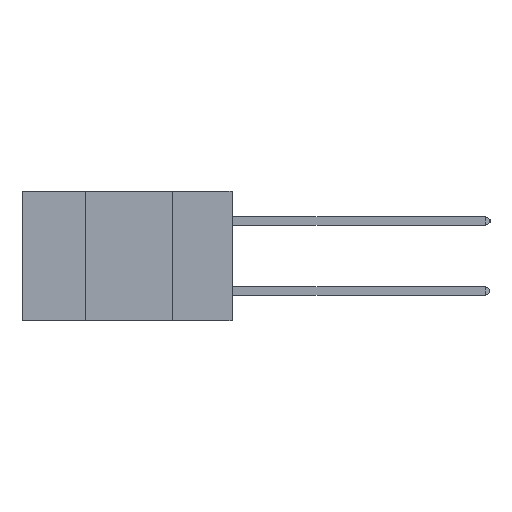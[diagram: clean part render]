
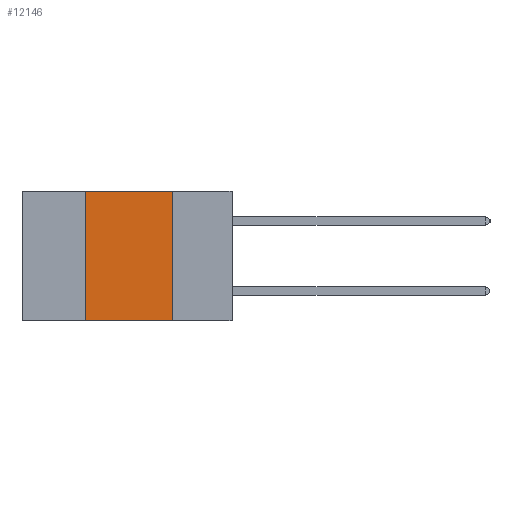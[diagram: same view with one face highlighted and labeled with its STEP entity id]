
A CAD part, left-side view. The second image highlights one B-rep face of the part: STEP entity #12146.
In plain terms, the highlighted planar face has unit normal (-1, 0, 0).
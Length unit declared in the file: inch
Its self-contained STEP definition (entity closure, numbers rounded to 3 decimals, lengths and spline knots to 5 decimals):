
#1187 = VECTOR ( 'NONE', #5307, 39.37008 ) ;
#1372 = ORIENTED_EDGE ( 'NONE', *, *, #10143, .F. ) ;
#1518 = EDGE_LOOP ( 'NONE', ( #11757, #1372, #4082, #6726 ) ) ;
#1736 = DIRECTION ( 'NONE',  ( 1., 0., 0. ) ) ;
#1915 = VERTEX_POINT ( 'NONE', #3395 ) ;
#2028 = CARTESIAN_POINT ( 'NONE',  ( 0., 0.6, -0.37 ) ) ;
#2125 = EDGE_CURVE ( 'NONE', #6571, #8781, #4030, .T. ) ;
#2692 = CARTESIAN_POINT ( 'NONE',  ( 0., 0.17, -0.37 ) ) ;
#2729 = DIRECTION ( 'NONE',  ( 0., 0., 1. ) ) ;
#2883 = CARTESIAN_POINT ( 'NONE',  ( 0., 0.42, 0. ) ) ;
#3104 = AXIS2_PLACEMENT_3D ( 'NONE', #11746, #1736, #8810 ) ;
#3157 = CARTESIAN_POINT ( 'NONE',  ( 0., 0.17, 0. ) ) ;
#3200 = DIRECTION ( 'NONE',  ( 0., 0., -1. ) ) ;
#3228 = CARTESIAN_POINT ( 'NONE',  ( 0., 0.42, -0.37 ) ) ;
#3395 = CARTESIAN_POINT ( 'NONE',  ( 0., 0.42, 0. ) ) ;
#3723 = VECTOR ( 'NONE', #11494, 39.37008 ) ;
#3902 = LINE ( 'NONE', #2883, #11580 ) ;
#4030 = LINE ( 'NONE', #2028, #3723 ) ;
#4082 = ORIENTED_EDGE ( 'NONE', *, *, #5499, .F. ) ;
#5307 = DIRECTION ( 'NONE',  ( 0., -1., 0. ) ) ;
#5499 = EDGE_CURVE ( 'NONE', #6571, #1915, #3902, .T. ) ;
#6571 = VERTEX_POINT ( 'NONE', #3228 ) ;
#6576 = EDGE_CURVE ( 'NONE', #10217, #8781, #7137, .T. ) ;
#6726 = ORIENTED_EDGE ( 'NONE', *, *, #2125, .T. ) ;
#7137 = LINE ( 'NONE', #3157, #12441 ) ;
#8446 = CARTESIAN_POINT ( 'NONE',  ( 0., 0.17, 0. ) ) ;
#8781 = VERTEX_POINT ( 'NONE', #2692 ) ;
#8810 = DIRECTION ( 'NONE',  ( 0., 0., -1. ) ) ;
#9276 = LINE ( 'NONE', #11321, #1187 ) ;
#9526 = FACE_OUTER_BOUND ( 'NONE', #1518, .T. ) ;
#9760 = PLANE ( 'NONE',  #3104 ) ;
#10143 = EDGE_CURVE ( 'NONE', #1915, #10217, #9276, .T. ) ;
#10217 = VERTEX_POINT ( 'NONE', #8446 ) ;
#11321 = CARTESIAN_POINT ( 'NONE',  ( 0., 0.6, 0. ) ) ;
#11494 = DIRECTION ( 'NONE',  ( 0., -1., 0. ) ) ;
#11580 = VECTOR ( 'NONE', #2729, 39.37008 ) ;
#11746 = CARTESIAN_POINT ( 'NONE',  ( 0., 0.6, 0. ) ) ;
#11757 = ORIENTED_EDGE ( 'NONE', *, *, #6576, .F. ) ;
#12146 = ADVANCED_FACE ( 'NONE', ( #9526 ), #9760, .F. ) ;
#12441 = VECTOR ( 'NONE', #3200, 39.37008 ) ;
